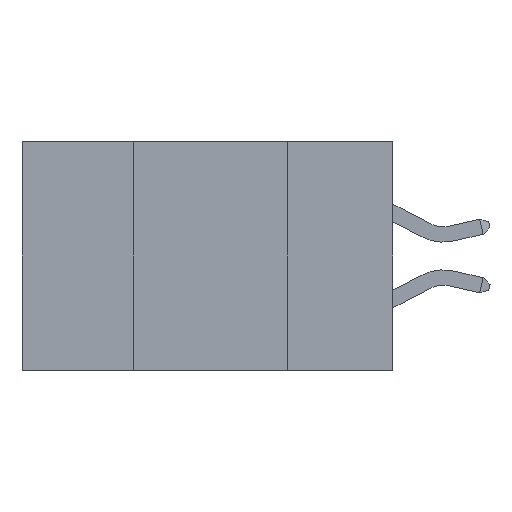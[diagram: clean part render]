
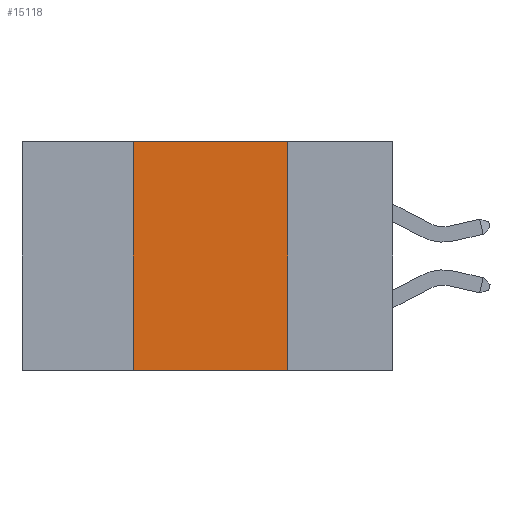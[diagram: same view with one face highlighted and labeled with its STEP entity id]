
A CAD part, left-side view. The second image highlights one B-rep face of the part: STEP entity #15118.
In plain terms, the highlighted planar face has unit normal (-1, 0, 0).
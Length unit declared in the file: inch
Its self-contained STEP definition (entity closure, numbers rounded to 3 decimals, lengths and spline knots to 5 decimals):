
#22 = DIRECTION ( 'NONE',  ( 0., 0., -1. ) ) ;
#1216 = CARTESIAN_POINT ( 'NONE',  ( 0., 0.42, 0. ) ) ;
#2538 = EDGE_CURVE ( 'NONE', #28802, #20552, #12757, .T. ) ;
#3236 = CARTESIAN_POINT ( 'NONE',  ( 0., 0.42, -0.37 ) ) ;
#3454 = CARTESIAN_POINT ( 'NONE',  ( 0., 0.42, 0. ) ) ;
#5378 = AXIS2_PLACEMENT_3D ( 'NONE', #5550, #22494, #7815 ) ;
#5550 = CARTESIAN_POINT ( 'NONE',  ( 0., 0.6, 0. ) ) ;
#6307 = VECTOR ( 'NONE', #30269, 39.37008 ) ;
#6596 = VECTOR ( 'NONE', #25081, 39.37008 ) ;
#7815 = DIRECTION ( 'NONE',  ( 0., 0., -1. ) ) ;
#7833 = FACE_OUTER_BOUND ( 'NONE', #15398, .T. ) ;
#9331 = ORIENTED_EDGE ( 'NONE', *, *, #18594, .F. ) ;
#9495 = ORIENTED_EDGE ( 'NONE', *, *, #29821, .F. ) ;
#9728 = CARTESIAN_POINT ( 'NONE',  ( 0., 0.6, 0. ) ) ;
#10320 = VERTEX_POINT ( 'NONE', #13158 ) ;
#10323 = PLANE ( 'NONE',  #5378 ) ;
#12276 = CARTESIAN_POINT ( 'NONE',  ( 0., 0.17, 0. ) ) ;
#12757 = LINE ( 'NONE', #1216, #6307 ) ;
#13158 = CARTESIAN_POINT ( 'NONE',  ( 0., 0.17, 0. ) ) ;
#14219 = LINE ( 'NONE', #12276, #27431 ) ;
#14794 = DIRECTION ( 'NONE',  ( 0., -1., 0. ) ) ;
#15049 = VERTEX_POINT ( 'NONE', #27432 ) ;
#15118 = ADVANCED_FACE ( 'NONE', ( #7833 ), #10323, .F. ) ;
#15398 = EDGE_LOOP ( 'NONE', ( #9495, #9331, #19590, #24019 ) ) ;
#15749 = EDGE_CURVE ( 'NONE', #28802, #15049, #28517, .T. ) ;
#18594 = EDGE_CURVE ( 'NONE', #20552, #10320, #22314, .T. ) ;
#19590 = ORIENTED_EDGE ( 'NONE', *, *, #2538, .F. ) ;
#20552 = VERTEX_POINT ( 'NONE', #3454 ) ;
#22314 = LINE ( 'NONE', #9728, #30961 ) ;
#22494 = DIRECTION ( 'NONE',  ( 1., 0., 0. ) ) ;
#22770 = CARTESIAN_POINT ( 'NONE',  ( 0., 0.6, -0.37 ) ) ;
#24019 = ORIENTED_EDGE ( 'NONE', *, *, #15749, .T. ) ;
#25081 = DIRECTION ( 'NONE',  ( 0., -1., 0. ) ) ;
#27431 = VECTOR ( 'NONE', #22, 39.37008 ) ;
#27432 = CARTESIAN_POINT ( 'NONE',  ( 0., 0.17, -0.37 ) ) ;
#28517 = LINE ( 'NONE', #22770, #6596 ) ;
#28802 = VERTEX_POINT ( 'NONE', #3236 ) ;
#29821 = EDGE_CURVE ( 'NONE', #10320, #15049, #14219, .T. ) ;
#30269 = DIRECTION ( 'NONE',  ( 0., 0., 1. ) ) ;
#30961 = VECTOR ( 'NONE', #14794, 39.37008 ) ;
